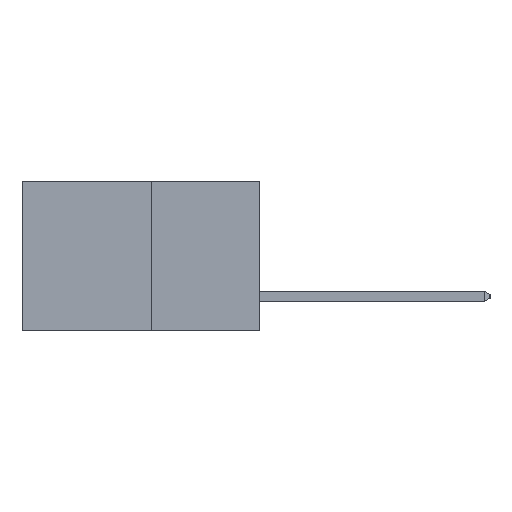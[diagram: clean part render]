
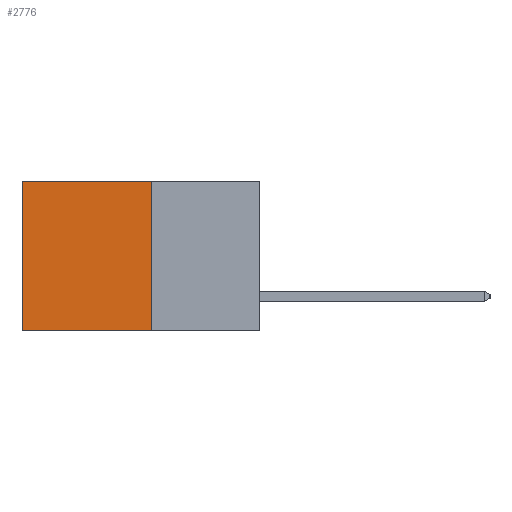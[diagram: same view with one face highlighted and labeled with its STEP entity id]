
A CAD part, left-side view. The second image highlights one B-rep face of the part: STEP entity #2776.
In plain terms, the highlighted planar face has unit normal (-1, 0, 0).
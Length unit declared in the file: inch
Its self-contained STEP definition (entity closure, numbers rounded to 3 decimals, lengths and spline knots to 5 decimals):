
#200 = ORIENTED_EDGE ( 'NONE', *, *, #331, .F. ) ;
#211 = LINE ( 'NONE', #6548, #3597 ) ;
#220 = EDGE_CURVE ( 'NONE', #2094, #4712, #5613, .T. ) ;
#331 = EDGE_CURVE ( 'NONE', #2094, #4279, #6528, .T. ) ;
#511 = CARTESIAN_POINT ( 'NONE',  ( 0.277, 0.59, 0. ) ) ;
#822 = LINE ( 'NONE', #1230, #5136 ) ;
#1063 = CARTESIAN_POINT ( 'NONE',  ( 0.277, 0.27, -0.37 ) ) ;
#1221 = EDGE_CURVE ( 'NONE', #4279, #3886, #822, .T. ) ;
#1230 = CARTESIAN_POINT ( 'NONE',  ( 0.277, 0.27, -0.37 ) ) ;
#1754 = DIRECTION ( 'NONE',  ( 0., 1., 0. ) ) ;
#1866 = ORIENTED_EDGE ( 'NONE', *, *, #220, .T. ) ;
#2094 = VERTEX_POINT ( 'NONE', #9046 ) ;
#2735 = CARTESIAN_POINT ( 'NONE',  ( 0.277, 0.27, -0.37 ) ) ;
#2776 = ADVANCED_FACE ( 'NONE', ( #4434 ), #5117, .F. ) ;
#3071 = EDGE_CURVE ( 'NONE', #4712, #3886, #211, .T. ) ;
#3306 = CARTESIAN_POINT ( 'NONE',  ( 0.277, 0.27, 0. ) ) ;
#3349 = ORIENTED_EDGE ( 'NONE', *, *, #1221, .F. ) ;
#3597 = VECTOR ( 'NONE', #6647, 39.37008 ) ;
#3607 = VECTOR ( 'NONE', #1754, 39.37008 ) ;
#3886 = VERTEX_POINT ( 'NONE', #4679 ) ;
#4068 = DIRECTION ( 'NONE',  ( 0., 0., -1. ) ) ;
#4083 = DIRECTION ( 'NONE',  ( 1., 0., 0. ) ) ;
#4279 = VERTEX_POINT ( 'NONE', #2735 ) ;
#4434 = FACE_OUTER_BOUND ( 'NONE', #6467, .T. ) ;
#4676 = VECTOR ( 'NONE', #5687, 39.37008 ) ;
#4679 = CARTESIAN_POINT ( 'NONE',  ( 0.277, 0.59, -0.37 ) ) ;
#4712 = VERTEX_POINT ( 'NONE', #511 ) ;
#5117 = PLANE ( 'NONE',  #7327 ) ;
#5136 = VECTOR ( 'NONE', #8176, 39.37008 ) ;
#5613 = LINE ( 'NONE', #3306, #3607 ) ;
#5687 = DIRECTION ( 'NONE',  ( 0., 0., -1. ) ) ;
#6467 = EDGE_LOOP ( 'NONE', ( #7791, #3349, #200, #1866 ) ) ;
#6528 = LINE ( 'NONE', #6648, #4676 ) ;
#6548 = CARTESIAN_POINT ( 'NONE',  ( 0.277, 0.59, -0.37 ) ) ;
#6647 = DIRECTION ( 'NONE',  ( 0., 0., -1. ) ) ;
#6648 = CARTESIAN_POINT ( 'NONE',  ( 0.277, 0.27, -0.37 ) ) ;
#7327 = AXIS2_PLACEMENT_3D ( 'NONE', #1063, #4083, #4068 ) ;
#7791 = ORIENTED_EDGE ( 'NONE', *, *, #3071, .T. ) ;
#8176 = DIRECTION ( 'NONE',  ( 0., 1., 0. ) ) ;
#9046 = CARTESIAN_POINT ( 'NONE',  ( 0.277, 0.27, 0. ) ) ;
